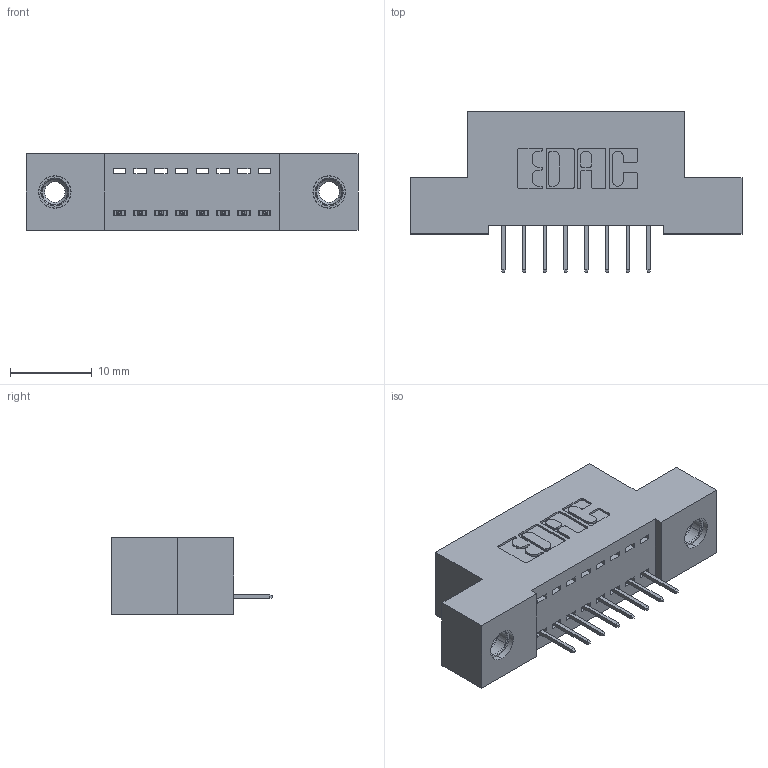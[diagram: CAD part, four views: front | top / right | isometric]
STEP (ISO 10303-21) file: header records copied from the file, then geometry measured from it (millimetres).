
FILE_DESCRIPTION (( 'STEP AP203' ), '1' );
FILE_NAME ('392-008-524-107.STEP', '2019-10-04T23:50:27', ( '' ), ( '' ), 'SwSTEP 2.0', 'SolidWorks 2016', '' );
FILE_SCHEMA (( 'CONFIG_CONTROL_DESIGN' ));
Length unit declared in the file: inch
Products named in the file (4): 345-292-001_345-293-124; 345-250-001_345-250-005-103; 392-008-524-107; 342 Part_TI
Assembly tree (11 placements, depth 2):
  392-008-524-107
    342 Part_TI
    345-292-001_345-293-124  x8
    345-250-001_345-250-005-103  x2
Bounding box: 40.64 x 19.69 x 9.4 mm (x, y, z)
Volume: 3393.8 mm3; surface area: 4282.8 mm2
Topology: 11 solids, 11 shells, 666 faces, 1875 edges, 1210 vertices
Faces by surface type: plane 482, cylinder 168, cone 12, torus 4
Entity records: 10416 total; most frequent: CARTESIAN_POINT 1781, ORIENTED_EDGE 1718, DIRECTION 1605, EDGE_CURVE 859, LINE 715, VECTOR 715, VERTEX_POINT 564, AXIS2_PLACEMENT_3D 445
